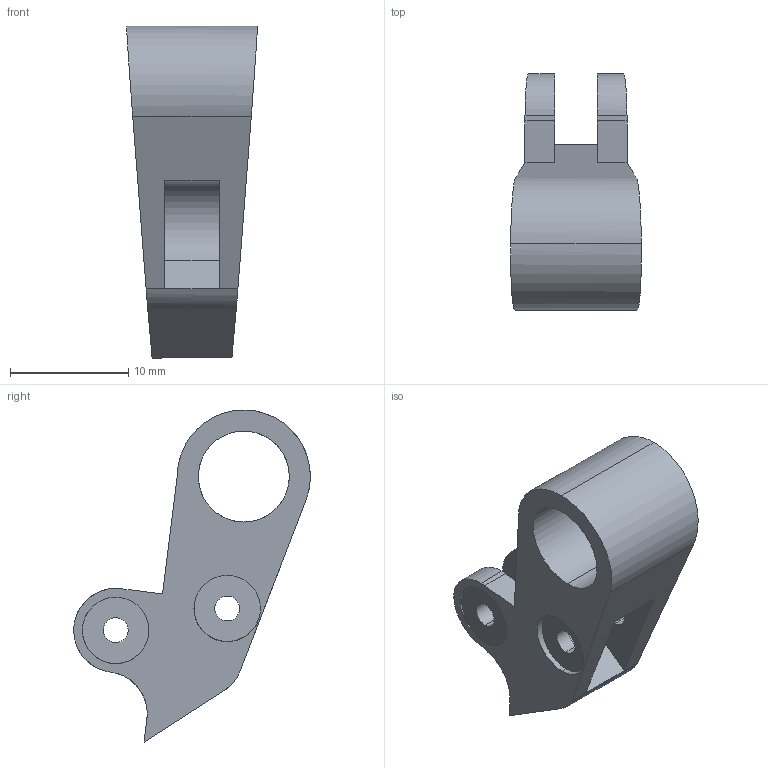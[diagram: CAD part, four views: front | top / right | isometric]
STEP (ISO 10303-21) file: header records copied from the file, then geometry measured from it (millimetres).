
FILE_DESCRIPTION (( 'STEP AP203' ), '1' );
FILE_NAME ('Sear.STEP', '2013-09-22T12:20:08', ( '' ), ( '' ), 'SwSTEP 2.0', 'SolidWorks 2013', '' );
FILE_SCHEMA (( 'CONFIG_CONTROL_DESIGN' ));
Length unit declared in the file: millimetre
Products named in the file (1): Sear
Bounding box: 11.06 x 20 x 28.07 mm (x, y, z)
Volume: 1573.7 mm3; surface area: 1647.3 mm2
Topology: 1 solids, 1 shells, 49 faces, 127 edges, 84 vertices
Faces by surface type: cylinder 31, plane 18
Entity records: 1598 total; most frequent: CARTESIAN_POINT 339, ORIENTED_EDGE 254, DIRECTION 237, EDGE_CURVE 127, AXIS2_PLACEMENT_3D 86, VERTEX_POINT 84, VECTOR 65, LINE 65
